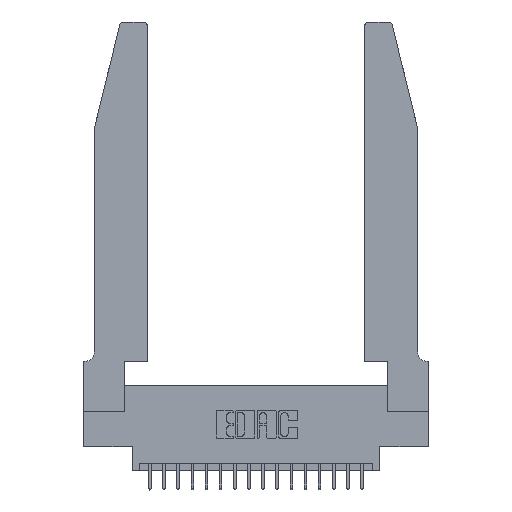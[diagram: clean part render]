
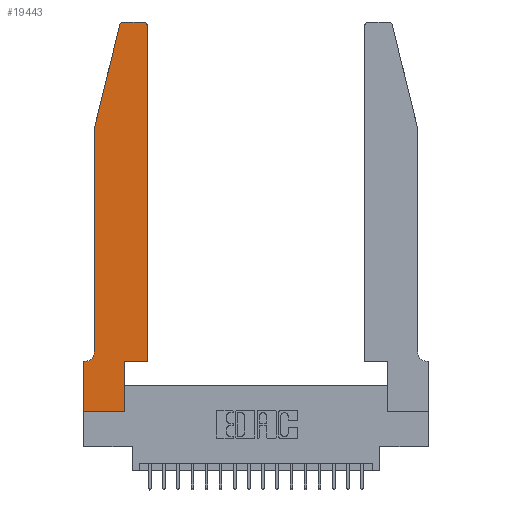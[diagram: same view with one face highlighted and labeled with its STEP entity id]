
A CAD part, top view. The second image highlights one B-rep face of the part: STEP entity #19443.
In plain terms, the highlighted planar face has unit normal (0, 0, 1).
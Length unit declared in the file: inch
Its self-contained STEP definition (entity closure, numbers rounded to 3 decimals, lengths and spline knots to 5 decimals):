
#121 = CARTESIAN_POINT ( 'NONE',  ( 0., 0., 0.37 ) ) ;
#345 = EDGE_CURVE ( 'NONE', #5795, #6889, #6387, .T. ) ;
#404 = DIRECTION ( 'NONE',  ( 0., 0., -1. ) ) ;
#479 = EDGE_LOOP ( 'NONE', ( #2135, #14222, #7454, #13696, #8276, #20921, #9905, #20132, #12979, #6256, #15079, #3477 ) ) ;
#767 = CARTESIAN_POINT ( 'NONE',  ( 0., 0.35, 0.37 ) ) ;
#868 = EDGE_CURVE ( 'NONE', #3397, #11478, #17784, .T. ) ;
#1014 = VECTOR ( 'NONE', #14605, 39.37008 ) ;
#1069 = CARTESIAN_POINT ( 'NONE',  ( 0.0755, 2., 0.37 ) ) ;
#1101 = LINE ( 'NONE', #4201, #14553 ) ;
#1650 = EDGE_CURVE ( 'NONE', #11608, #3397, #8326, .T. ) ;
#1730 = EDGE_CURVE ( 'NONE', #11478, #8915, #12293, .T. ) ;
#1746 = CARTESIAN_POINT ( 'NONE',  ( 0.4205, 2.72, 0.37 ) ) ;
#1946 = VECTOR ( 'NONE', #12685, 39.37008 ) ;
#2135 = ORIENTED_EDGE ( 'NONE', *, *, #16505, .T. ) ;
#2504 = DIRECTION ( 'NONE',  ( 1., 0., 0. ) ) ;
#2507 = LINE ( 'NONE', #2706, #14953 ) ;
#2706 = CARTESIAN_POINT ( 'NONE',  ( 0.2865, 0.35, 0.37 ) ) ;
#2969 = EDGE_CURVE ( 'NONE', #6889, #16135, #18217, .T. ) ;
#3066 = EDGE_CURVE ( 'NONE', #8962, #11608, #4173, .T. ) ;
#3397 = VERTEX_POINT ( 'NONE', #15118 ) ;
#3477 = ORIENTED_EDGE ( 'NONE', *, *, #8270, .T. ) ;
#3530 = DIRECTION ( 'NONE',  ( 0., 0., 1. ) ) ;
#3702 = VERTEX_POINT ( 'NONE', #13135 ) ;
#4056 = CARTESIAN_POINT ( 'NONE',  ( 0.0755, 0.35, 0.37 ) ) ;
#4173 = LINE ( 'NONE', #1069, #20904 ) ;
#4201 = CARTESIAN_POINT ( 'NONE',  ( 0., 0., 0.37 ) ) ;
#4401 = CIRCLE ( 'NONE', #13943, 0.03 ) ;
#4884 = CARTESIAN_POINT ( 'NONE',  ( 0.0755, 2., 0.37 ) ) ;
#5170 = DIRECTION ( 'NONE',  ( 0., 0., 1. ) ) ;
#5490 = VECTOR ( 'NONE', #13972, 39.37008 ) ;
#5795 = VERTEX_POINT ( 'NONE', #20820 ) ;
#5860 = DIRECTION ( 'NONE',  ( 1., 0., 0. ) ) ;
#6152 = CARTESIAN_POINT ( 'NONE',  ( 0.2605, 2.75, 0.37 ) ) ;
#6256 = ORIENTED_EDGE ( 'NONE', *, *, #345, .T. ) ;
#6384 = CIRCLE ( 'NONE', #10833, 0.03 ) ;
#6387 = LINE ( 'NONE', #9816, #1014 ) ;
#6788 = CARTESIAN_POINT ( 'NONE',  ( 0.4505, 0.35, 0.37 ) ) ;
#6889 = VERTEX_POINT ( 'NONE', #6788 ) ;
#7454 = ORIENTED_EDGE ( 'NONE', *, *, #3066, .T. ) ;
#7540 = VECTOR ( 'NONE', #20165, 39.37008 ) ;
#8270 = EDGE_CURVE ( 'NONE', #16135, #15524, #6384, .T. ) ;
#8276 = ORIENTED_EDGE ( 'NONE', *, *, #868, .T. ) ;
#8326 = LINE ( 'NONE', #11757, #13593 ) ;
#8915 = VERTEX_POINT ( 'NONE', #767 ) ;
#8962 = VERTEX_POINT ( 'NONE', #10693 ) ;
#9190 = AXIS2_PLACEMENT_3D ( 'NONE', #13962, #20438, #5860 ) ;
#9816 = CARTESIAN_POINT ( 'NONE',  ( 0.4505, 0.35, 0.37 ) ) ;
#9905 = ORIENTED_EDGE ( 'NONE', *, *, #14148, .T. ) ;
#9988 = EDGE_CURVE ( 'NONE', #15783, #8962, #4401, .T. ) ;
#10045 = DIRECTION ( 'NONE',  ( 1., 0., 0. ) ) ;
#10048 = VECTOR ( 'NONE', #12086, 39.37008 ) ;
#10250 = DIRECTION ( 'NONE',  ( 0., -1., 0. ) ) ;
#10693 = CARTESIAN_POINT ( 'NONE',  ( 0.25487, 2.72718, 0.37 ) ) ;
#10697 = AXIS2_PLACEMENT_3D ( 'NONE', #14689, #404, #15004 ) ;
#10833 = AXIS2_PLACEMENT_3D ( 'NONE', #1746, #5170, #16331 ) ;
#11478 = VERTEX_POINT ( 'NONE', #15154 ) ;
#11608 = VERTEX_POINT ( 'NONE', #4884 ) ;
#11757 = CARTESIAN_POINT ( 'NONE',  ( 0.0755, 2., 0.37 ) ) ;
#12040 = CARTESIAN_POINT ( 'NONE',  ( 0.284, 2.75, 0.37 ) ) ;
#12086 = DIRECTION ( 'NONE',  ( 0., 1., 0. ) ) ;
#12293 = LINE ( 'NONE', #4056, #5490 ) ;
#12520 = LINE ( 'NONE', #13693, #7540 ) ;
#12685 = DIRECTION ( 'NONE',  ( -1., 0., 0. ) ) ;
#12979 = ORIENTED_EDGE ( 'NONE', *, *, #18689, .T. ) ;
#13135 = CARTESIAN_POINT ( 'NONE',  ( 0.2865, 0., 0.37 ) ) ;
#13253 = CARTESIAN_POINT ( 'NONE',  ( 0.284, 2.72, 0.37 ) ) ;
#13365 = PLANE ( 'NONE',  #9190 ) ;
#13459 = FACE_OUTER_BOUND ( 'NONE', #479, .T. ) ;
#13593 = VECTOR ( 'NONE', #10250, 39.37008 ) ;
#13693 = CARTESIAN_POINT ( 'NONE',  ( 0., 0., 0.37 ) ) ;
#13696 = ORIENTED_EDGE ( 'NONE', *, *, #1650, .T. ) ;
#13869 = DIRECTION ( 'NONE',  ( -0.239, -0.971, 0. ) ) ;
#13943 = AXIS2_PLACEMENT_3D ( 'NONE', #13253, #3530, #10045 ) ;
#13962 = CARTESIAN_POINT ( 'NONE',  ( 0., 0.35, 0.37 ) ) ;
#13972 = DIRECTION ( 'NONE',  ( -1., 0., 0. ) ) ;
#14148 = EDGE_CURVE ( 'NONE', #8915, #19220, #12520, .T. ) ;
#14214 = DIRECTION ( 'NONE',  ( 0., 1., 0. ) ) ;
#14222 = ORIENTED_EDGE ( 'NONE', *, *, #9988, .T. ) ;
#14553 = VECTOR ( 'NONE', #2504, 39.37008 ) ;
#14605 = DIRECTION ( 'NONE',  ( 1., 0., 0. ) ) ;
#14689 = CARTESIAN_POINT ( 'NONE',  ( 0.0055, 0.42, 0.37 ) ) ;
#14953 = VECTOR ( 'NONE', #14214, 39.37008 ) ;
#15004 = DIRECTION ( 'NONE',  ( -1., 0., 0. ) ) ;
#15079 = ORIENTED_EDGE ( 'NONE', *, *, #2969, .T. ) ;
#15118 = CARTESIAN_POINT ( 'NONE',  ( 0.0755, 0.42, 0.37 ) ) ;
#15154 = CARTESIAN_POINT ( 'NONE',  ( 0.0055, 0.35, 0.37 ) ) ;
#15367 = CARTESIAN_POINT ( 'NONE',  ( 0.4505, 2.72, 0.37 ) ) ;
#15524 = VERTEX_POINT ( 'NONE', #17442 ) ;
#15783 = VERTEX_POINT ( 'NONE', #12040 ) ;
#16135 = VERTEX_POINT ( 'NONE', #15367 ) ;
#16331 = DIRECTION ( 'NONE',  ( 1., 0., 0. ) ) ;
#16505 = EDGE_CURVE ( 'NONE', #15524, #15783, #17130, .T. ) ;
#16513 = CARTESIAN_POINT ( 'NONE',  ( 0.4505, 0.35, 0.37 ) ) ;
#17130 = LINE ( 'NONE', #6152, #1946 ) ;
#17442 = CARTESIAN_POINT ( 'NONE',  ( 0.4205, 2.75, 0.37 ) ) ;
#17473 = EDGE_CURVE ( 'NONE', #19220, #3702, #1101, .T. ) ;
#17784 = CIRCLE ( 'NONE', #10697, 0.07 ) ;
#18217 = LINE ( 'NONE', #16513, #10048 ) ;
#18689 = EDGE_CURVE ( 'NONE', #3702, #5795, #2507, .T. ) ;
#19220 = VERTEX_POINT ( 'NONE', #121 ) ;
#19443 = ADVANCED_FACE ( 'NONE', ( #13459 ), #13365, .T. ) ;
#20132 = ORIENTED_EDGE ( 'NONE', *, *, #17473, .T. ) ;
#20165 = DIRECTION ( 'NONE',  ( 0., -1., 0. ) ) ;
#20438 = DIRECTION ( 'NONE',  ( 0., 0., 1. ) ) ;
#20820 = CARTESIAN_POINT ( 'NONE',  ( 0.2865, 0.35, 0.37 ) ) ;
#20904 = VECTOR ( 'NONE', #13869, 39.37008 ) ;
#20921 = ORIENTED_EDGE ( 'NONE', *, *, #1730, .T. ) ;
